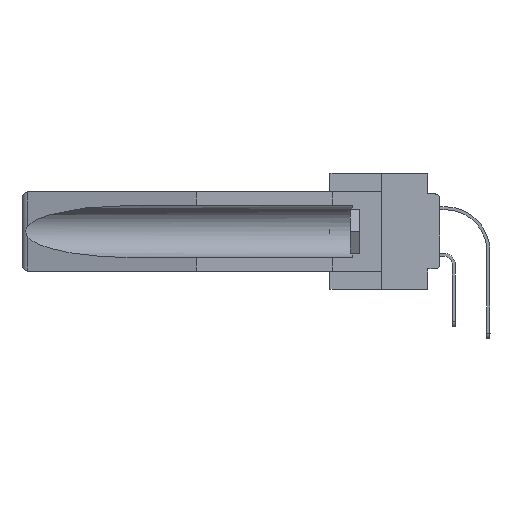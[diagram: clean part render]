
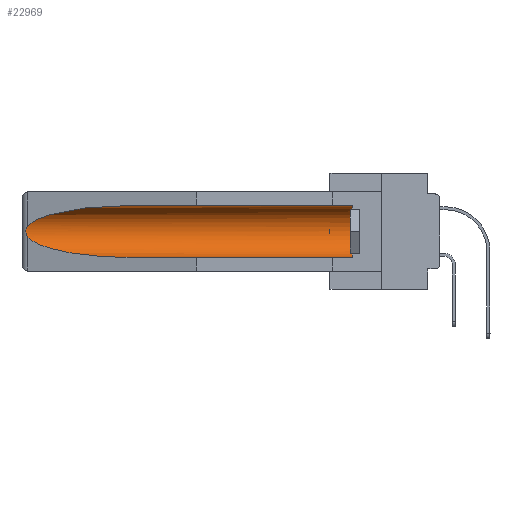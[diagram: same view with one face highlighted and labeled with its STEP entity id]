
A CAD part, left-side view. The second image highlights one B-rep face of the part: STEP entity #22969.
In plain terms, the highlighted cylindrical face has radius 2.857 mm (diameter 5.715 mm), a partial arc.
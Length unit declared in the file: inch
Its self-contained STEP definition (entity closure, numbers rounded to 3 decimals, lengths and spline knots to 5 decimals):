
#254 = CARTESIAN_POINT ( 'NONE',  ( 0.155, 0.126, -0.284 ) ) ;
#704 = ORIENTED_EDGE ( 'NONE', *, *, #2965, .T. ) ;
#1784 = B_SPLINE_CURVE_WITH_KNOTS ( 'NONE', 3,
 ( #1925, #21307, #27277, #8531, #17487, #37055, #34282, #30249, #34472, #11739 ),
 .UNSPECIFIED., .F., .F.,
 ( 4, 2, 2, 2, 4 ),
 ( 0., 0.00029, 0.00058, 0.00087, 0.00117 ),
 .UNSPECIFIED. ) ;
#1925 = CARTESIAN_POINT ( 'NONE',  ( 0.26537, 1.52718, -0.14972 ) ) ;
#2582 = CARTESIAN_POINT ( 'NONE',  ( 0.26537, 1.52718, -0.14972 ) ) ;
#2583 = LINE ( 'NONE', #15592, #19686 ) ;
#2669 = ORIENTED_EDGE ( 'NONE', *, *, #40495, .F. ) ;
#2740 = VERTEX_POINT ( 'NONE', #4747 ) ;
#2965 = EDGE_CURVE ( 'NONE', #2740, #18048, #15886, .T. ) ;
#3641 = CARTESIAN_POINT ( 'NONE',  ( 0.155, 1.07973, -0.284 ) ) ;
#4747 = CARTESIAN_POINT ( 'NONE',  ( 0.26537, 1.52718, -0.19328 ) ) ;
#6901 = EDGE_LOOP ( 'NONE', ( #22913, #39272, #704, #2669, #39037, #9442 ) ) ;
#8531 = CARTESIAN_POINT ( 'NONE',  ( 0.2673, 1.5327, -0.16383 ) ) ;
#9442 = ORIENTED_EDGE ( 'NONE', *, *, #31498, .T. ) ;
#9636 = EDGE_CURVE ( 'NONE', #13248, #26896, #26089, .T. ) ;
#10235 = CARTESIAN_POINT ( 'NONE',  ( 0.21114, 1.30732, -0.284 ) ) ;
#11739 = CARTESIAN_POINT ( 'NONE',  ( 0.26537, 1.52718, -0.19328 ) ) ;
#12362 = VERTEX_POINT ( 'NONE', #26536 ) ;
#12584 = DIRECTION ( 'NONE',  ( 0., 1., 0. ) ) ;
#13248 = VERTEX_POINT ( 'NONE', #254 ) ;
#15592 = CARTESIAN_POINT ( 'NONE',  ( 0.155, -0.30754, -0.059 ) ) ;
#15886 =( BOUNDED_CURVE ( )  B_SPLINE_CURVE ( 3, ( #29403, #39599, #10235, #3641 ),
 .UNSPECIFIED., .F., .F. ) 
 B_SPLINE_CURVE_WITH_KNOTS ( ( 4, 4 ),
 ( 0.1948, 1.5708 ),
 .UNSPECIFIED. ) 
 CURVE ( )  GEOMETRIC_REPRESENTATION_ITEM ( )  RATIONAL_B_SPLINE_CURVE ( ( 1., 0.848, 0.848, 1. ) ) 
 REPRESENTATION_ITEM ( '' )  );
#16652 = VERTEX_POINT ( 'NONE', #2582 ) ;
#17487 = CARTESIAN_POINT ( 'NONE',  ( 0.2675, 1.53308, -0.16763 ) ) ;
#18048 = VERTEX_POINT ( 'NONE', #38545 ) ;
#18561 = CARTESIAN_POINT ( 'NONE',  ( 0.155, 0.126, -0.1715 ) ) ;
#18598 = EDGE_CURVE ( 'NONE', #12362, #16652, #18612, .T. ) ;
#18612 =( BOUNDED_CURVE ( )  B_SPLINE_CURVE ( 3, ( #33159, #23408, #29348, #29135 ),
 .UNSPECIFIED., .F., .F. ) 
 B_SPLINE_CURVE_WITH_KNOTS ( ( 4, 4 ),
 ( 4.71239, 6.08839 ),
 .UNSPECIFIED. ) 
 CURVE ( )  GEOMETRIC_REPRESENTATION_ITEM ( )  RATIONAL_B_SPLINE_CURVE ( ( 1., 0.848, 0.848, 1. ) ) 
 REPRESENTATION_ITEM ( '' )  );
#18668 = AXIS2_PLACEMENT_3D ( 'NONE', #32757, #12584, #19388 ) ;
#19388 = DIRECTION ( 'NONE',  ( 0., 0., 1. ) ) ;
#19606 = EDGE_CURVE ( 'NONE', #16652, #2740, #1784, .T. ) ;
#19686 = VECTOR ( 'NONE', #28552, 39.37008 ) ;
#19788 = FACE_OUTER_BOUND ( 'NONE', #6901, .T. ) ;
#19938 = AXIS2_PLACEMENT_3D ( 'NONE', #18561, #34300, #41300 ) ;
#21307 = CARTESIAN_POINT ( 'NONE',  ( 0.26597, 1.52961, -0.15275 ) ) ;
#22913 = ORIENTED_EDGE ( 'NONE', *, *, #18598, .T. ) ;
#22969 = ADVANCED_FACE ( 'NONE', ( #19788 ), #38941, .F. ) ;
#23408 = CARTESIAN_POINT ( 'NONE',  ( 0.21114, 1.30732, -0.059 ) ) ;
#26089 = CIRCLE ( 'NONE', #19938, 0.1125 ) ;
#26536 = CARTESIAN_POINT ( 'NONE',  ( 0.155, 1.07973, -0.059 ) ) ;
#26896 = VERTEX_POINT ( 'NONE', #29255 ) ;
#27277 = CARTESIAN_POINT ( 'NONE',  ( 0.26654, 1.53092, -0.15636 ) ) ;
#27321 = DIRECTION ( 'NONE',  ( 0., 1., 0. ) ) ;
#27458 = VECTOR ( 'NONE', #27321, 39.37008 ) ;
#28552 = DIRECTION ( 'NONE',  ( 0., 1., 0. ) ) ;
#29135 = CARTESIAN_POINT ( 'NONE',  ( 0.26537, 1.52718, -0.14972 ) ) ;
#29255 = CARTESIAN_POINT ( 'NONE',  ( 0.155, 0.126, -0.059 ) ) ;
#29348 = CARTESIAN_POINT ( 'NONE',  ( 0.25451, 1.48313, -0.09465 ) ) ;
#29403 = CARTESIAN_POINT ( 'NONE',  ( 0.26537, 1.52718, -0.19328 ) ) ;
#30249 = CARTESIAN_POINT ( 'NONE',  ( 0.26655, 1.53094, -0.18657 ) ) ;
#31498 = EDGE_CURVE ( 'NONE', #26896, #12362, #2583, .T. ) ;
#32757 = CARTESIAN_POINT ( 'NONE',  ( 0.155, -0.30754, -0.1715 ) ) ;
#33159 = CARTESIAN_POINT ( 'NONE',  ( 0.155, 1.07973, -0.059 ) ) ;
#33472 = LINE ( 'NONE', #34109, #27458 ) ;
#34109 = CARTESIAN_POINT ( 'NONE',  ( 0.155, -0.30754, -0.284 ) ) ;
#34282 = CARTESIAN_POINT ( 'NONE',  ( 0.2673, 1.53269, -0.17917 ) ) ;
#34300 = DIRECTION ( 'NONE',  ( 0., -1., 0. ) ) ;
#34472 = CARTESIAN_POINT ( 'NONE',  ( 0.26597, 1.5296, -0.19026 ) ) ;
#37055 = CARTESIAN_POINT ( 'NONE',  ( 0.2675, 1.53308, -0.17534 ) ) ;
#38545 = CARTESIAN_POINT ( 'NONE',  ( 0.155, 1.07973, -0.284 ) ) ;
#38941 = CYLINDRICAL_SURFACE ( 'NONE', #18668, 0.1125 ) ;
#39037 = ORIENTED_EDGE ( 'NONE', *, *, #9636, .T. ) ;
#39272 = ORIENTED_EDGE ( 'NONE', *, *, #19606, .T. ) ;
#39599 = CARTESIAN_POINT ( 'NONE',  ( 0.25451, 1.48313, -0.24835 ) ) ;
#40495 = EDGE_CURVE ( 'NONE', #13248, #18048, #33472, .T. ) ;
#41300 = DIRECTION ( 'NONE',  ( 0., 0., 1. ) ) ;
